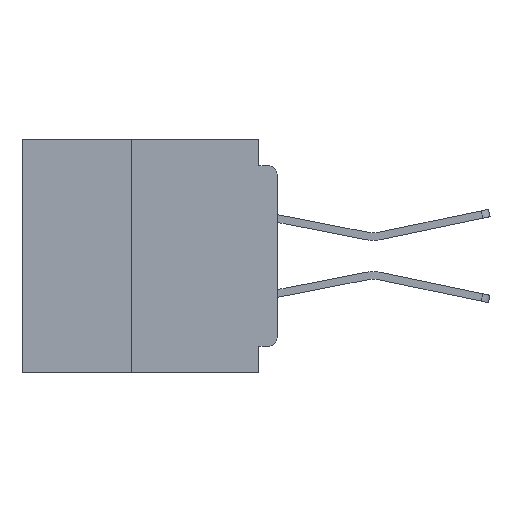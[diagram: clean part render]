
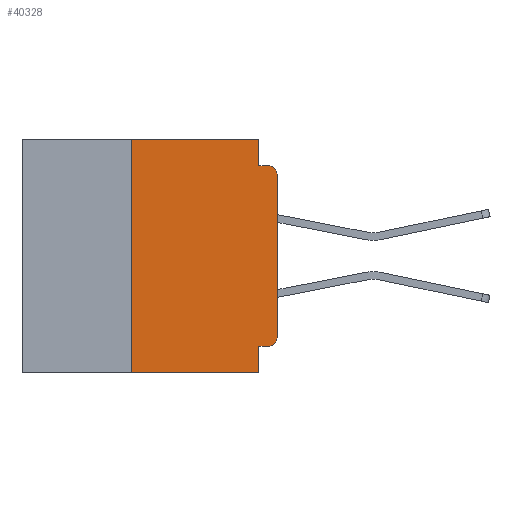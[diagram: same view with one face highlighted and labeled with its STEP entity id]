
A CAD part, left-side view. The second image highlights one B-rep face of the part: STEP entity #40328.
In plain terms, the highlighted planar face has unit normal (-1, 0, 0).
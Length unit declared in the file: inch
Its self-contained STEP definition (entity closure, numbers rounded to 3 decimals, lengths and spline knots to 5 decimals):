
#202 = VERTEX_POINT ( 'NONE', #19936 ) ;
#232 = VECTOR ( 'NONE', #31652, 39.37008 ) ;
#963 = EDGE_CURVE ( 'NONE', #6610, #16333, #15518, .T. ) ;
#1799 = CARTESIAN_POINT ( 'NONE',  ( 0., 0.015, -0.06 ) ) ;
#2733 = DIRECTION ( 'NONE',  ( 0., 1., 0. ) ) ;
#3221 = CARTESIAN_POINT ( 'NONE',  ( 0., 0.25, -0.4 ) ) ;
#3397 = LINE ( 'NONE', #49724, #13439 ) ;
#4130 = EDGE_CURVE ( 'NONE', #31411, #37013, #48646, .T. ) ;
#5559 = EDGE_CURVE ( 'NONE', #16810, #31411, #30026, .T. ) ;
#6398 = AXIS2_PLACEMENT_3D ( 'NONE', #21483, #50766, #25704 ) ;
#6545 = VECTOR ( 'NONE', #2733, 39.37008 ) ;
#6610 = VERTEX_POINT ( 'NONE', #51524 ) ;
#7303 = VERTEX_POINT ( 'NONE', #51977 ) ;
#8050 = FACE_OUTER_BOUND ( 'NONE', #16297, .T. ) ;
#9733 = DIRECTION ( 'NONE',  ( 1., 0., 0. ) ) ;
#10004 = DIRECTION ( 'NONE',  ( 0., 0., -1. ) ) ;
#10437 = ORIENTED_EDGE ( 'NONE', *, *, #12646, .F. ) ;
#10548 = CARTESIAN_POINT ( 'NONE',  ( 0., 0.25, -0.4 ) ) ;
#10568 = DIRECTION ( 'NONE',  ( -1., 0., 0. ) ) ;
#10643 = DIRECTION ( 'NONE',  ( 0., 0., -1. ) ) ;
#11406 = VECTOR ( 'NONE', #10004, 39.37008 ) ;
#11839 = CARTESIAN_POINT ( 'NONE',  ( 0., 0.25, 0. ) ) ;
#12421 = EDGE_CURVE ( 'NONE', #7303, #16333, #3397, .T. ) ;
#12646 = EDGE_CURVE ( 'NONE', #37013, #7303, #12759, .T. ) ;
#12759 = LINE ( 'NONE', #31005, #11406 ) ;
#13061 = EDGE_CURVE ( 'NONE', #27753, #202, #25249, .T. ) ;
#13439 = VECTOR ( 'NONE', #20416, 39.37008 ) ;
#13517 = DIRECTION ( 'NONE',  ( 0., 0., 1. ) ) ;
#15158 = VECTOR ( 'NONE', #22507, 39.37008 ) ;
#15518 = CIRCLE ( 'NONE', #53189, 0.015 ) ;
#16297 = EDGE_LOOP ( 'NONE', ( #48564, #38692, #20385, #10437, #25674, #50555, #51813, #30888, #43320, #44642 ) ) ;
#16333 = VERTEX_POINT ( 'NONE', #37965 ) ;
#16810 = VERTEX_POINT ( 'NONE', #3221 ) ;
#17052 = DIRECTION ( 'NONE',  ( 0., 0., -1. ) ) ;
#17163 = AXIS2_PLACEMENT_3D ( 'NONE', #34938, #9733, #39139 ) ;
#17611 = CARTESIAN_POINT ( 'NONE',  ( 0., 0., 0. ) ) ;
#18215 = CARTESIAN_POINT ( 'NONE',  ( 0., 0.031, 0. ) ) ;
#18302 = CARTESIAN_POINT ( 'NONE',  ( 0., 0.437, 0. ) ) ;
#19030 = EDGE_CURVE ( 'NONE', #25206, #6610, #38869, .T. ) ;
#19613 = CARTESIAN_POINT ( 'NONE',  ( 0., 0., -0.34 ) ) ;
#19936 = CARTESIAN_POINT ( 'NONE',  ( 0., 0.031, -0.4 ) ) ;
#20385 = ORIENTED_EDGE ( 'NONE', *, *, #12421, .F. ) ;
#20416 = DIRECTION ( 'NONE',  ( 0., -1., 0. ) ) ;
#21483 = CARTESIAN_POINT ( 'NONE',  ( 0., 0.015, -0.34 ) ) ;
#22507 = DIRECTION ( 'NONE',  ( 0., -1., 0. ) ) ;
#25206 = VERTEX_POINT ( 'NONE', #19613 ) ;
#25249 = LINE ( 'NONE', #42140, #35018 ) ;
#25674 = ORIENTED_EDGE ( 'NONE', *, *, #4130, .F. ) ;
#25704 = DIRECTION ( 'NONE',  ( 0., 0., -1. ) ) ;
#27753 = VERTEX_POINT ( 'NONE', #34872 ) ;
#29081 = LINE ( 'NONE', #53183, #6545 ) ;
#29642 = CARTESIAN_POINT ( 'NONE',  ( 0., 0.015, -0.355 ) ) ;
#30026 = LINE ( 'NONE', #10548, #50978 ) ;
#30311 = VERTEX_POINT ( 'NONE', #29642 ) ;
#30888 = ORIENTED_EDGE ( 'NONE', *, *, #13061, .F. ) ;
#31005 = CARTESIAN_POINT ( 'NONE',  ( 0., 0.031, 0. ) ) ;
#31411 = VERTEX_POINT ( 'NONE', #11839 ) ;
#31467 = CARTESIAN_POINT ( 'NONE',  ( 0., 0.437, -0.4 ) ) ;
#31652 = DIRECTION ( 'NONE',  ( 0., -1., 0. ) ) ;
#32920 = CIRCLE ( 'NONE', #6398, 0.015 ) ;
#34000 = LINE ( 'NONE', #31467, #232 ) ;
#34872 = CARTESIAN_POINT ( 'NONE',  ( 0., 0.031, -0.355 ) ) ;
#34938 = CARTESIAN_POINT ( 'NONE',  ( 0., 0.437, 0. ) ) ;
#35018 = VECTOR ( 'NONE', #17052, 39.37008 ) ;
#35311 = EDGE_CURVE ( 'NONE', #30311, #27753, #29081, .T. ) ;
#37013 = VERTEX_POINT ( 'NONE', #18215 ) ;
#37965 = CARTESIAN_POINT ( 'NONE',  ( 0., 0.015, -0.045 ) ) ;
#38692 = ORIENTED_EDGE ( 'NONE', *, *, #963, .T. ) ;
#38869 = LINE ( 'NONE', #17611, #47389 ) ;
#39139 = DIRECTION ( 'NONE',  ( 0., 0., -1. ) ) ;
#40328 = ADVANCED_FACE ( 'NONE', ( #8050 ), #51595, .F. ) ;
#42140 = CARTESIAN_POINT ( 'NONE',  ( 0., 0.031, -0.4 ) ) ;
#42786 = EDGE_CURVE ( 'NONE', #16810, #202, #34000, .T. ) ;
#43320 = ORIENTED_EDGE ( 'NONE', *, *, #35311, .F. ) ;
#44642 = ORIENTED_EDGE ( 'NONE', *, *, #46477, .T. ) ;
#46477 = EDGE_CURVE ( 'NONE', #30311, #25206, #32920, .T. ) ;
#47389 = VECTOR ( 'NONE', #13517, 39.37008 ) ;
#48564 = ORIENTED_EDGE ( 'NONE', *, *, #19030, .T. ) ;
#48646 = LINE ( 'NONE', #18302, #15158 ) ;
#49724 = CARTESIAN_POINT ( 'NONE',  ( 0., 0., -0.045 ) ) ;
#50555 = ORIENTED_EDGE ( 'NONE', *, *, #5559, .F. ) ;
#50766 = DIRECTION ( 'NONE',  ( -1., 0., 0. ) ) ;
#50978 = VECTOR ( 'NONE', #52559, 39.37008 ) ;
#51524 = CARTESIAN_POINT ( 'NONE',  ( 0., 0., -0.06 ) ) ;
#51595 = PLANE ( 'NONE',  #17163 ) ;
#51813 = ORIENTED_EDGE ( 'NONE', *, *, #42786, .T. ) ;
#51977 = CARTESIAN_POINT ( 'NONE',  ( 0., 0.031, -0.045 ) ) ;
#52559 = DIRECTION ( 'NONE',  ( 0., 0., 1. ) ) ;
#53183 = CARTESIAN_POINT ( 'NONE',  ( 0., 0., -0.355 ) ) ;
#53189 = AXIS2_PLACEMENT_3D ( 'NONE', #1799, #10568, #10643 ) ;
